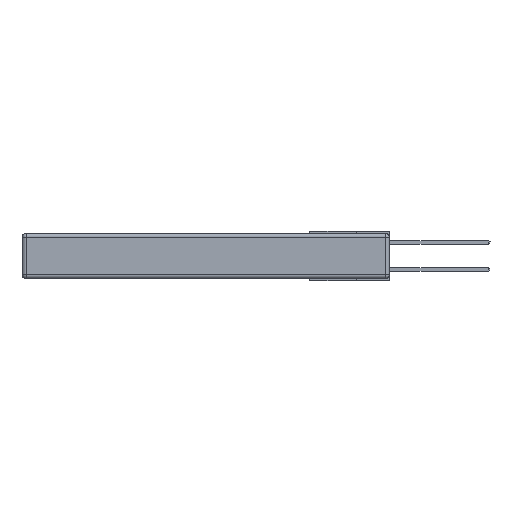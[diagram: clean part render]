
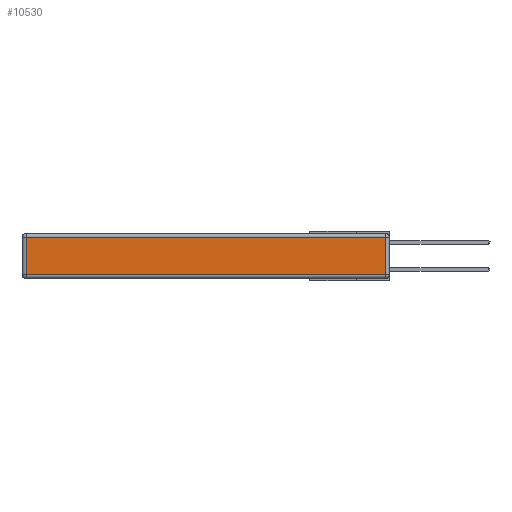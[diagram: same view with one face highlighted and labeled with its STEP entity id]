
A CAD part, left-side view. The second image highlights one B-rep face of the part: STEP entity #10530.
In plain terms, the highlighted planar face has unit normal (-1, 0, 0).
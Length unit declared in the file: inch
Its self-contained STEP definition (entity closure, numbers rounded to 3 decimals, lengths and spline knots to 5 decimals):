
#52 = VERTEX_POINT ( 'NONE', #14789 ) ;
#443 = DIRECTION ( 'NONE',  ( 0., -1., 0. ) ) ;
#1756 = EDGE_CURVE ( 'NONE', #20683, #52, #20471, .T. ) ;
#3016 = ORIENTED_EDGE ( 'NONE', *, *, #5550, .T. ) ;
#3448 = CARTESIAN_POINT ( 'NONE',  ( 0., 0.03, -0.343 ) ) ;
#3492 = VECTOR ( 'NONE', #7757, 39.37008 ) ;
#4482 = CARTESIAN_POINT ( 'NONE',  ( 0., 2.72, -0.313 ) ) ;
#5094 = VECTOR ( 'NONE', #443, 39.37008 ) ;
#5422 = VERTEX_POINT ( 'NONE', #19047 ) ;
#5550 = EDGE_CURVE ( 'NONE', #52, #5422, #11209, .T. ) ;
#6475 = VECTOR ( 'NONE', #12316, 39.37008 ) ;
#6982 = CARTESIAN_POINT ( 'NONE',  ( 0., 0., -0.343 ) ) ;
#7735 = CARTESIAN_POINT ( 'NONE',  ( 0., 2.72, -0.03 ) ) ;
#7757 = DIRECTION ( 'NONE',  ( 0., 0., -1. ) ) ;
#8166 = AXIS2_PLACEMENT_3D ( 'NONE', #6982, #17418, #12200 ) ;
#8919 = VECTOR ( 'NONE', #20730, 39.37008 ) ;
#9443 = ORIENTED_EDGE ( 'NONE', *, *, #1756, .T. ) ;
#10530 = ADVANCED_FACE ( 'NONE', ( #21880 ), #17644, .T. ) ;
#10824 = ORIENTED_EDGE ( 'NONE', *, *, #13115, .T. ) ;
#11155 = LINE ( 'NONE', #13459, #8919 ) ;
#11209 = LINE ( 'NONE', #3448, #6475 ) ;
#12200 = DIRECTION ( 'NONE',  ( 0., 0., 1. ) ) ;
#12316 = DIRECTION ( 'NONE',  ( 0., 0., 1. ) ) ;
#13115 = EDGE_CURVE ( 'NONE', #5422, #14814, #11155, .T. ) ;
#13459 = CARTESIAN_POINT ( 'NONE',  ( 0., 2.75, -0.03 ) ) ;
#14403 = ORIENTED_EDGE ( 'NONE', *, *, #18279, .T. ) ;
#14481 = CARTESIAN_POINT ( 'NONE',  ( 0., 0., -0.313 ) ) ;
#14789 = CARTESIAN_POINT ( 'NONE',  ( 0., 0.03, -0.313 ) ) ;
#14814 = VERTEX_POINT ( 'NONE', #7735 ) ;
#16975 = EDGE_LOOP ( 'NONE', ( #9443, #3016, #10824, #14403 ) ) ;
#17418 = DIRECTION ( 'NONE',  ( -1., 0., 0. ) ) ;
#17644 = PLANE ( 'NONE',  #8166 ) ;
#18279 = EDGE_CURVE ( 'NONE', #14814, #20683, #20543, .T. ) ;
#18448 = CARTESIAN_POINT ( 'NONE',  ( 0., 2.72, -0.343 ) ) ;
#19047 = CARTESIAN_POINT ( 'NONE',  ( 0., 0.03, -0.03 ) ) ;
#20471 = LINE ( 'NONE', #14481, #5094 ) ;
#20543 = LINE ( 'NONE', #18448, #3492 ) ;
#20683 = VERTEX_POINT ( 'NONE', #4482 ) ;
#20730 = DIRECTION ( 'NONE',  ( 0., 1., 0. ) ) ;
#21880 = FACE_OUTER_BOUND ( 'NONE', #16975, .T. ) ;
